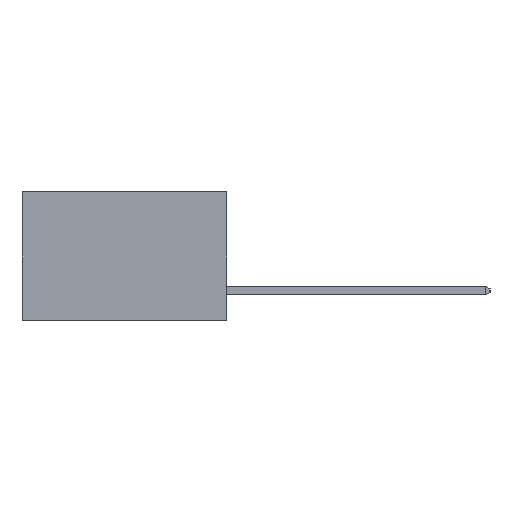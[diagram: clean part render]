
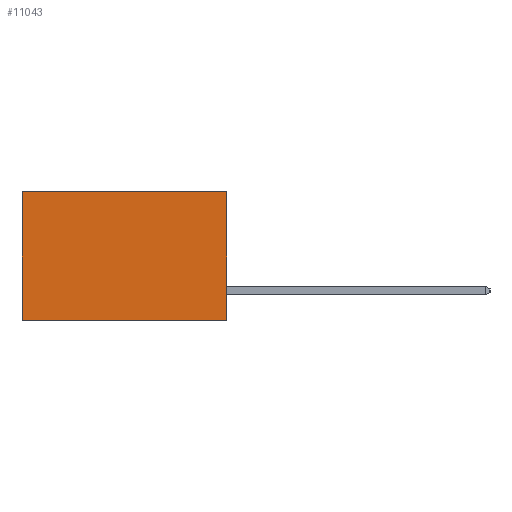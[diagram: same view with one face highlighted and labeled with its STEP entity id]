
A CAD part, left-side view. The second image highlights one B-rep face of the part: STEP entity #11043.
In plain terms, the highlighted planar face has unit normal (-1, 0, 0).
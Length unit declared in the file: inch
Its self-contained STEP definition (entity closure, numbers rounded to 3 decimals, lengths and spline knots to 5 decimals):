
#216 = CARTESIAN_POINT ( 'NONE',  ( 0.277, 0., -0.37 ) ) ;
#326 = VECTOR ( 'NONE', #11362, 39.37008 ) ;
#1375 = AXIS2_PLACEMENT_3D ( 'NONE', #3936, #19567, #7890 ) ;
#2434 = VERTEX_POINT ( 'NONE', #13645 ) ;
#3011 = EDGE_CURVE ( 'NONE', #24166, #15169, #21671, .T. ) ;
#3936 = CARTESIAN_POINT ( 'NONE',  ( 0.277, 0., -0.37 ) ) ;
#4626 = CARTESIAN_POINT ( 'NONE',  ( 0.277, 0.59, -0.37 ) ) ;
#4747 = ORIENTED_EDGE ( 'NONE', *, *, #16454, .T. ) ;
#5800 = VECTOR ( 'NONE', #6880, 39.37008 ) ;
#6880 = DIRECTION ( 'NONE',  ( 0., 1., 0. ) ) ;
#7089 = VECTOR ( 'NONE', #14232, 39.37008 ) ;
#7890 = DIRECTION ( 'NONE',  ( 0., 0., -1. ) ) ;
#11043 = ADVANCED_FACE ( 'NONE', ( #16905 ), #17625, .F. ) ;
#11362 = DIRECTION ( 'NONE',  ( 0., 1., 0. ) ) ;
#11390 = LINE ( 'NONE', #13221, #326 ) ;
#11856 = EDGE_CURVE ( 'NONE', #14947, #2434, #22611, .T. ) ;
#12331 = CARTESIAN_POINT ( 'NONE',  ( 0.277, 0., -0.37 ) ) ;
#12739 = EDGE_CURVE ( 'NONE', #2434, #15169, #16189, .T. ) ;
#12760 = EDGE_LOOP ( 'NONE', ( #24496, #14795, #15126, #4747 ) ) ;
#13221 = CARTESIAN_POINT ( 'NONE',  ( 0.277, 0., 0. ) ) ;
#13645 = CARTESIAN_POINT ( 'NONE',  ( 0.277, 0., -0.37 ) ) ;
#14232 = DIRECTION ( 'NONE',  ( 0., 0., -1. ) ) ;
#14795 = ORIENTED_EDGE ( 'NONE', *, *, #12739, .F. ) ;
#14947 = VERTEX_POINT ( 'NONE', #19408 ) ;
#15126 = ORIENTED_EDGE ( 'NONE', *, *, #11856, .F. ) ;
#15169 = VERTEX_POINT ( 'NONE', #4626 ) ;
#15327 = CARTESIAN_POINT ( 'NONE',  ( 0.277, 0.59, -0.37 ) ) ;
#15911 = VECTOR ( 'NONE', #19372, 39.37008 ) ;
#16189 = LINE ( 'NONE', #216, #5800 ) ;
#16454 = EDGE_CURVE ( 'NONE', #14947, #24166, #11390, .T. ) ;
#16905 = FACE_OUTER_BOUND ( 'NONE', #12760, .T. ) ;
#17625 = PLANE ( 'NONE',  #1375 ) ;
#19372 = DIRECTION ( 'NONE',  ( 0., 0., -1. ) ) ;
#19408 = CARTESIAN_POINT ( 'NONE',  ( 0.277, 0., 0. ) ) ;
#19567 = DIRECTION ( 'NONE',  ( 1., 0., 0. ) ) ;
#21671 = LINE ( 'NONE', #15327, #15911 ) ;
#22611 = LINE ( 'NONE', #12331, #7089 ) ;
#22835 = CARTESIAN_POINT ( 'NONE',  ( 0.277, 0.59, 0. ) ) ;
#24166 = VERTEX_POINT ( 'NONE', #22835 ) ;
#24496 = ORIENTED_EDGE ( 'NONE', *, *, #3011, .T. ) ;
